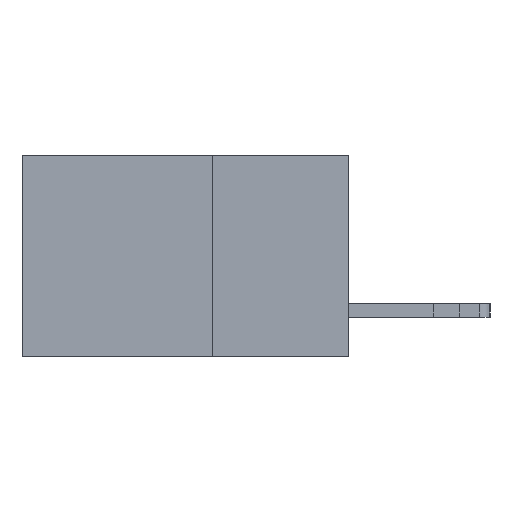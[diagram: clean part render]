
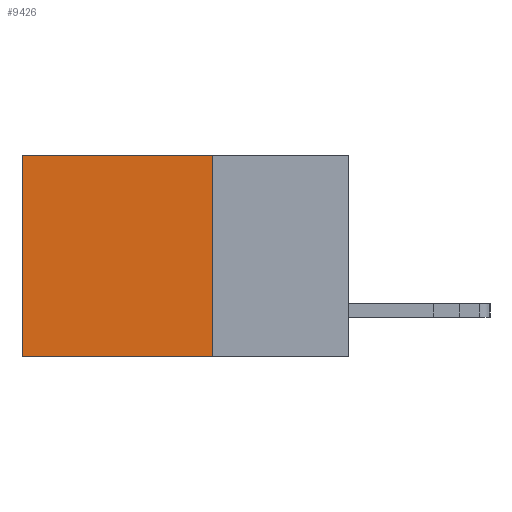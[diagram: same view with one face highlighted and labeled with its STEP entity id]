
A CAD part, left-side view. The second image highlights one B-rep face of the part: STEP entity #9426.
In plain terms, the highlighted planar face has unit normal (-1, 0, 0).
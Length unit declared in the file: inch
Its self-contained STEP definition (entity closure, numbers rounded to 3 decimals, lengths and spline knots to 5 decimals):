
#252 = DIRECTION ( 'NONE',  ( 0., 1., 0. ) ) ;
#282 = CARTESIAN_POINT ( 'NONE',  ( 0.298, 0.25, -0.37 ) ) ;
#1981 = CARTESIAN_POINT ( 'NONE',  ( 0.298, 0.25, 0. ) ) ;
#2429 = VERTEX_POINT ( 'NONE', #6493 ) ;
#3596 = DIRECTION ( 'NONE',  ( 0., 1., 0. ) ) ;
#3604 = VECTOR ( 'NONE', #8565, 39.37008 ) ;
#3805 = LINE ( 'NONE', #1981, #16095 ) ;
#4331 = FACE_OUTER_BOUND ( 'NONE', #14835, .T. ) ;
#5800 = VECTOR ( 'NONE', #252, 39.37008 ) ;
#6344 = ORIENTED_EDGE ( 'NONE', *, *, #18484, .T. ) ;
#6493 = CARTESIAN_POINT ( 'NONE',  ( 0.298, 0.6, 0. ) ) ;
#6605 = ORIENTED_EDGE ( 'NONE', *, *, #9100, .F. ) ;
#7045 = CARTESIAN_POINT ( 'NONE',  ( 0.298, 0.25, -0.37 ) ) ;
#7687 = CARTESIAN_POINT ( 'NONE',  ( 0.298, 0.6, -0.37 ) ) ;
#8149 = EDGE_CURVE ( 'NONE', #18813, #19975, #20092, .T. ) ;
#8565 = DIRECTION ( 'NONE',  ( 0., 0., -1. ) ) ;
#8568 = CARTESIAN_POINT ( 'NONE',  ( 0.298, 0.25, 0. ) ) ;
#8789 = DIRECTION ( 'NONE',  ( 0., 0., -1. ) ) ;
#9100 = EDGE_CURVE ( 'NONE', #19975, #16597, #10632, .T. ) ;
#9426 = ADVANCED_FACE ( 'NONE', ( #4331 ), #10687, .F. ) ;
#9770 = LINE ( 'NONE', #18749, #13024 ) ;
#10337 = DIRECTION ( 'NONE',  ( 1., 0., 0. ) ) ;
#10629 = CARTESIAN_POINT ( 'NONE',  ( 0.298, 0.25, 0. ) ) ;
#10632 = LINE ( 'NONE', #282, #5800 ) ;
#10687 = PLANE ( 'NONE',  #15811 ) ;
#10765 = DIRECTION ( 'NONE',  ( 0., 0., -1. ) ) ;
#13024 = VECTOR ( 'NONE', #10765, 39.37008 ) ;
#14040 = ORIENTED_EDGE ( 'NONE', *, *, #15374, .T. ) ;
#14835 = EDGE_LOOP ( 'NONE', ( #6344, #6605, #17605, #14040 ) ) ;
#15374 = EDGE_CURVE ( 'NONE', #18813, #2429, #3805, .T. ) ;
#15811 = AXIS2_PLACEMENT_3D ( 'NONE', #10629, #10337, #8789 ) ;
#16095 = VECTOR ( 'NONE', #3596, 39.37008 ) ;
#16597 = VERTEX_POINT ( 'NONE', #7687 ) ;
#16850 = CARTESIAN_POINT ( 'NONE',  ( 0.298, 0.25, 0. ) ) ;
#17605 = ORIENTED_EDGE ( 'NONE', *, *, #8149, .F. ) ;
#18484 = EDGE_CURVE ( 'NONE', #2429, #16597, #9770, .T. ) ;
#18749 = CARTESIAN_POINT ( 'NONE',  ( 0.298, 0.6, 0. ) ) ;
#18813 = VERTEX_POINT ( 'NONE', #16850 ) ;
#19975 = VERTEX_POINT ( 'NONE', #7045 ) ;
#20092 = LINE ( 'NONE', #8568, #3604 ) ;
